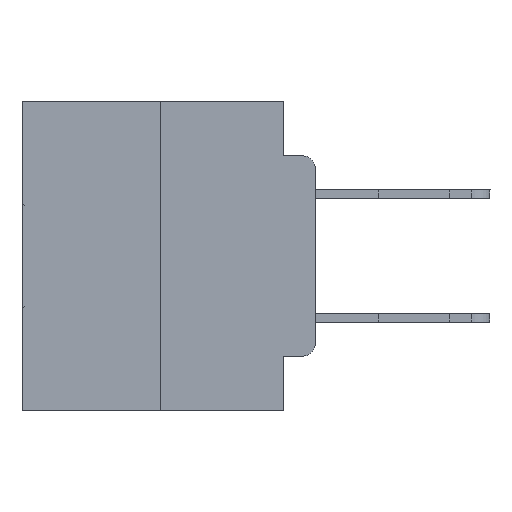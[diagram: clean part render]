
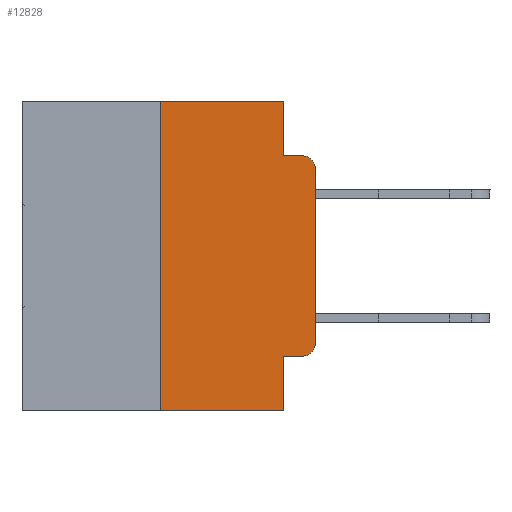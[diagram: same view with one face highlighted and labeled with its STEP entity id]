
A CAD part, left-side view. The second image highlights one B-rep face of the part: STEP entity #12828.
In plain terms, the highlighted planar face has unit normal (-1, 0, 0).
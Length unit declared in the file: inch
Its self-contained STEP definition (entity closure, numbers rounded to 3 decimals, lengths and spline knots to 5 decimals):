
#167 = ORIENTED_EDGE ( 'NONE', *, *, #14909, .T. ) ;
#332 = DIRECTION ( 'NONE',  ( 0., 0., -1. ) ) ;
#1049 = VERTEX_POINT ( 'NONE', #22942 ) ;
#1307 = VERTEX_POINT ( 'NONE', #16906 ) ;
#1340 = EDGE_LOOP ( 'NONE', ( #15520, #18249, #27589, #13326, #28985, #8899, #26668, #2354, #167, #16684 ) ) ;
#1691 = CARTESIAN_POINT ( 'NONE',  ( 0., 0., 0. ) ) ;
#2199 = VERTEX_POINT ( 'NONE', #17874 ) ;
#2354 = ORIENTED_EDGE ( 'NONE', *, *, #8391, .F. ) ;
#2370 = VECTOR ( 'NONE', #21095, 39.37008 ) ;
#2375 = DIRECTION ( 'NONE',  ( 0., 0., -1. ) ) ;
#2552 = VECTOR ( 'NONE', #332, 39.37008 ) ;
#2632 = DIRECTION ( 'NONE',  ( -1., 0., 0. ) ) ;
#2774 = CARTESIAN_POINT ( 'NONE',  ( 0., 0.25, 0. ) ) ;
#3297 = VERTEX_POINT ( 'NONE', #8675 ) ;
#3434 = VERTEX_POINT ( 'NONE', #7278 ) ;
#3441 = EDGE_CURVE ( 'NONE', #1049, #8470, #4109, .T. ) ;
#4109 = CIRCLE ( 'NONE', #16556, 0.02 ) ;
#4482 = LINE ( 'NONE', #13195, #22750 ) ;
#4829 = LINE ( 'NONE', #9066, #2552 ) ;
#5536 = CARTESIAN_POINT ( 'NONE',  ( 0., 0.051, -0.0885 ) ) ;
#6599 = VERTEX_POINT ( 'NONE', #26488 ) ;
#6804 = CARTESIAN_POINT ( 'NONE',  ( 0., 0.051, -0.4115 ) ) ;
#7278 = CARTESIAN_POINT ( 'NONE',  ( 0., 0.051, -0.4115 ) ) ;
#7453 = EDGE_CURVE ( 'NONE', #20673, #1049, #10536, .T. ) ;
#7916 = CARTESIAN_POINT ( 'NONE',  ( 0., 0., -0.3915 ) ) ;
#8391 = EDGE_CURVE ( 'NONE', #3434, #1307, #27243, .T. ) ;
#8427 = CARTESIAN_POINT ( 'NONE',  ( 0., 0.25, -0.5 ) ) ;
#8439 = EDGE_CURVE ( 'NONE', #2199, #6599, #4829, .T. ) ;
#8470 = VERTEX_POINT ( 'NONE', #18218 ) ;
#8675 = CARTESIAN_POINT ( 'NONE',  ( 0., 0.02, -0.4115 ) ) ;
#8899 = ORIENTED_EDGE ( 'NONE', *, *, #20958, .F. ) ;
#9066 = CARTESIAN_POINT ( 'NONE',  ( 0., 0.051, 0. ) ) ;
#9387 = EDGE_CURVE ( 'NONE', #14870, #2199, #4482, .T. ) ;
#10536 = LINE ( 'NONE', #1691, #24565 ) ;
#10596 = VERTEX_POINT ( 'NONE', #8427 ) ;
#11337 = AXIS2_PLACEMENT_3D ( 'NONE', #16037, #18433, #11659 ) ;
#11659 = DIRECTION ( 'NONE',  ( 0., 0., -1. ) ) ;
#12571 = DIRECTION ( 'NONE',  ( 0., -1., 0. ) ) ;
#12828 = ADVANCED_FACE ( 'NONE', ( #29278 ), #13634, .F. ) ;
#13195 = CARTESIAN_POINT ( 'NONE',  ( 0., 0.473, 0. ) ) ;
#13326 = ORIENTED_EDGE ( 'NONE', *, *, #8439, .F. ) ;
#13634 = PLANE ( 'NONE',  #18060 ) ;
#14694 = DIRECTION ( 'NONE',  ( 0., -1., 0. ) ) ;
#14870 = VERTEX_POINT ( 'NONE', #24090 ) ;
#14909 = EDGE_CURVE ( 'NONE', #3434, #3297, #29362, .T. ) ;
#15520 = ORIENTED_EDGE ( 'NONE', *, *, #7453, .T. ) ;
#16037 = CARTESIAN_POINT ( 'NONE',  ( 0., 0.02, -0.3915 ) ) ;
#16064 = EDGE_CURVE ( 'NONE', #3297, #20673, #21375, .T. ) ;
#16113 = DIRECTION ( 'NONE',  ( 0., 0., -1. ) ) ;
#16426 = DIRECTION ( 'NONE',  ( 0., 0., -1. ) ) ;
#16556 = AXIS2_PLACEMENT_3D ( 'NONE', #27437, #2632, #16426 ) ;
#16684 = ORIENTED_EDGE ( 'NONE', *, *, #16064, .T. ) ;
#16906 = CARTESIAN_POINT ( 'NONE',  ( 0., 0.051, -0.5 ) ) ;
#17426 = VECTOR ( 'NONE', #14694, 39.37008 ) ;
#17874 = CARTESIAN_POINT ( 'NONE',  ( 0., 0.051, 0. ) ) ;
#18060 = AXIS2_PLACEMENT_3D ( 'NONE', #24897, #25170, #2375 ) ;
#18218 = CARTESIAN_POINT ( 'NONE',  ( 0., 0.02, -0.0885 ) ) ;
#18249 = ORIENTED_EDGE ( 'NONE', *, *, #3441, .T. ) ;
#18433 = DIRECTION ( 'NONE',  ( -1., 0., 0. ) ) ;
#19042 = LINE ( 'NONE', #27926, #26823 ) ;
#20673 = VERTEX_POINT ( 'NONE', #7916 ) ;
#20913 = CARTESIAN_POINT ( 'NONE',  ( 0., 0.051, 0. ) ) ;
#20958 = EDGE_CURVE ( 'NONE', #10596, #14870, #23338, .T. ) ;
#21095 = DIRECTION ( 'NONE',  ( 0., 0., 1. ) ) ;
#21375 = CIRCLE ( 'NONE', #11337, 0.02 ) ;
#22239 = VECTOR ( 'NONE', #16113, 39.37008 ) ;
#22292 = DIRECTION ( 'NONE',  ( 0., -1., 0. ) ) ;
#22750 = VECTOR ( 'NONE', #27326, 39.37008 ) ;
#22759 = VECTOR ( 'NONE', #22292, 39.37008 ) ;
#22942 = CARTESIAN_POINT ( 'NONE',  ( 0., 0., -0.1085 ) ) ;
#23338 = LINE ( 'NONE', #2774, #2370 ) ;
#24090 = CARTESIAN_POINT ( 'NONE',  ( 0., 0.25, 0. ) ) ;
#24565 = VECTOR ( 'NONE', #28872, 39.37008 ) ;
#24897 = CARTESIAN_POINT ( 'NONE',  ( 0., 0.473, 0. ) ) ;
#25137 = EDGE_CURVE ( 'NONE', #6599, #8470, #26271, .T. ) ;
#25170 = DIRECTION ( 'NONE',  ( 1., 0., 0. ) ) ;
#26271 = LINE ( 'NONE', #5536, #17426 ) ;
#26488 = CARTESIAN_POINT ( 'NONE',  ( 0., 0.051, -0.0885 ) ) ;
#26668 = ORIENTED_EDGE ( 'NONE', *, *, #29102, .T. ) ;
#26823 = VECTOR ( 'NONE', #12571, 39.37008 ) ;
#27243 = LINE ( 'NONE', #20913, #22239 ) ;
#27326 = DIRECTION ( 'NONE',  ( 0., -1., 0. ) ) ;
#27437 = CARTESIAN_POINT ( 'NONE',  ( 0., 0.02, -0.1085 ) ) ;
#27589 = ORIENTED_EDGE ( 'NONE', *, *, #25137, .F. ) ;
#27926 = CARTESIAN_POINT ( 'NONE',  ( 0., 0.473, -0.5 ) ) ;
#28872 = DIRECTION ( 'NONE',  ( 0., 0., 1. ) ) ;
#28985 = ORIENTED_EDGE ( 'NONE', *, *, #9387, .F. ) ;
#29102 = EDGE_CURVE ( 'NONE', #10596, #1307, #19042, .T. ) ;
#29278 = FACE_OUTER_BOUND ( 'NONE', #1340, .T. ) ;
#29362 = LINE ( 'NONE', #6804, #22759 ) ;
